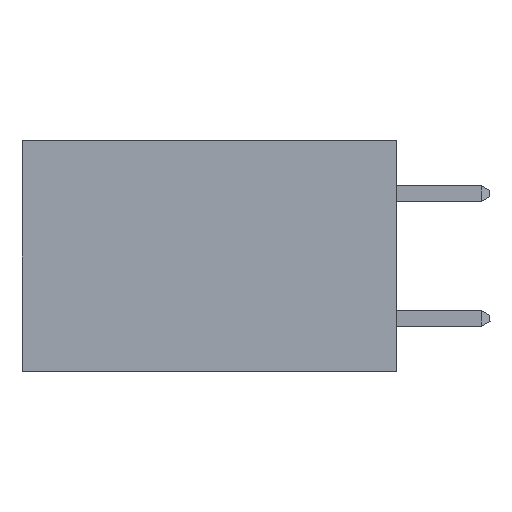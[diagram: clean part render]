
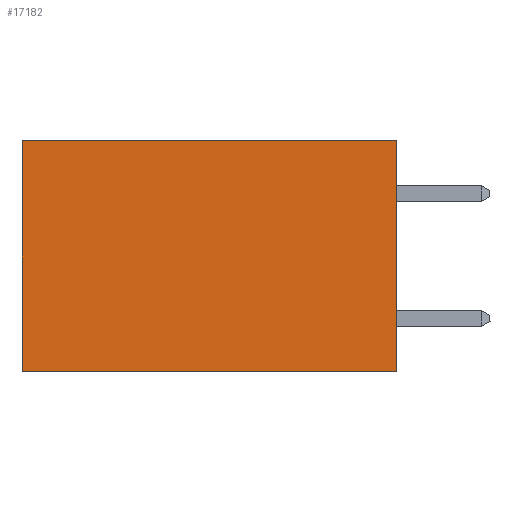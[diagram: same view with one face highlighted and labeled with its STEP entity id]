
A CAD part, left-side view. The second image highlights one B-rep face of the part: STEP entity #17182.
In plain terms, the highlighted planar face has unit normal (-1, 0, 0).
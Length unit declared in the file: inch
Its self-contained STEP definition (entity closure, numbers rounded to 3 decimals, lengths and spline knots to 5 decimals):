
#630 = CARTESIAN_POINT ( 'NONE',  ( 0.2615, 0., -0.37 ) ) ;
#731 = VERTEX_POINT ( 'NONE', #7052 ) ;
#1199 = VECTOR ( 'NONE', #23922, 39.37008 ) ;
#1243 = VECTOR ( 'NONE', #20489, 39.37008 ) ;
#2091 = VECTOR ( 'NONE', #19426, 39.37008 ) ;
#2312 = ORIENTED_EDGE ( 'NONE', *, *, #8100, .T. ) ;
#2783 = DIRECTION ( 'NONE',  ( 0., 0., -1. ) ) ;
#2934 = VERTEX_POINT ( 'NONE', #21387 ) ;
#3469 = FACE_OUTER_BOUND ( 'NONE', #14051, .T. ) ;
#3532 = EDGE_CURVE ( 'NONE', #2934, #8995, #16531, .T. ) ;
#3994 = ORIENTED_EDGE ( 'NONE', *, *, #4339, .F. ) ;
#4339 = EDGE_CURVE ( 'NONE', #12774, #2934, #7861, .T. ) ;
#6301 = LINE ( 'NONE', #15678, #1199 ) ;
#6353 = LINE ( 'NONE', #7872, #1243 ) ;
#6734 = AXIS2_PLACEMENT_3D ( 'NONE', #630, #15640, #2783 ) ;
#7052 = CARTESIAN_POINT ( 'NONE',  ( 0.2615, 0.6, 0. ) ) ;
#7861 = LINE ( 'NONE', #15227, #2091 ) ;
#7872 = CARTESIAN_POINT ( 'NONE',  ( 0.2615, 0., 0. ) ) ;
#8100 = EDGE_CURVE ( 'NONE', #731, #8995, #6301, .T. ) ;
#8995 = VERTEX_POINT ( 'NONE', #16260 ) ;
#9586 = ORIENTED_EDGE ( 'NONE', *, *, #12969, .T. ) ;
#12774 = VERTEX_POINT ( 'NONE', #23316 ) ;
#12909 = DIRECTION ( 'NONE',  ( 0., 1., 0. ) ) ;
#12969 = EDGE_CURVE ( 'NONE', #12774, #731, #6353, .T. ) ;
#13547 = PLANE ( 'NONE',  #6734 ) ;
#14051 = EDGE_LOOP ( 'NONE', ( #2312, #16010, #3994, #9586 ) ) ;
#15227 = CARTESIAN_POINT ( 'NONE',  ( 0.2615, 0., -0.37 ) ) ;
#15640 = DIRECTION ( 'NONE',  ( 1., 0., 0. ) ) ;
#15678 = CARTESIAN_POINT ( 'NONE',  ( 0.2615, 0.6, -0.37 ) ) ;
#15881 = VECTOR ( 'NONE', #12909, 39.37008 ) ;
#16010 = ORIENTED_EDGE ( 'NONE', *, *, #3532, .F. ) ;
#16260 = CARTESIAN_POINT ( 'NONE',  ( 0.2615, 0.6, -0.37 ) ) ;
#16531 = LINE ( 'NONE', #23265, #15881 ) ;
#17182 = ADVANCED_FACE ( 'NONE', ( #3469 ), #13547, .F. ) ;
#19426 = DIRECTION ( 'NONE',  ( 0., 0., -1. ) ) ;
#20489 = DIRECTION ( 'NONE',  ( 0., 1., 0. ) ) ;
#21387 = CARTESIAN_POINT ( 'NONE',  ( 0.2615, 0., -0.37 ) ) ;
#23265 = CARTESIAN_POINT ( 'NONE',  ( 0.2615, 0., -0.37 ) ) ;
#23316 = CARTESIAN_POINT ( 'NONE',  ( 0.2615, 0., 0. ) ) ;
#23922 = DIRECTION ( 'NONE',  ( 0., 0., -1. ) ) ;
